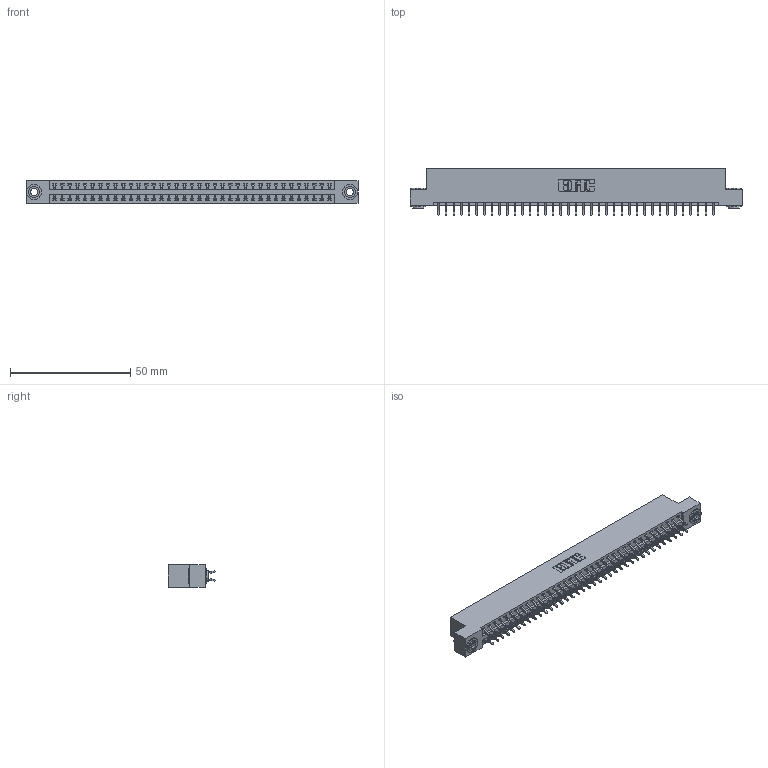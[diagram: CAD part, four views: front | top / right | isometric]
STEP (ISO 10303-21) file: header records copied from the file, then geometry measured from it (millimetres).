
FILE_DESCRIPTION (( 'STEP AP203' ), '1' );
FILE_NAME ('396-074-556-203.STEP', '2019-10-30T20:57:10', ( '' ), ( '' ), 'SwSTEP 2.0', 'SolidWorks 2016', '' );
FILE_SCHEMA (( 'CONFIG_CONTROL_DESIGN' ));
Length unit declared in the file: inch
Products named in the file (4): 396-074-556-203; 345-292-001_556 Tail; 345-250-002_345-250-002-102; 346 Part_Flush Mounting Lugs - 0.156 Dia-TH
Assembly tree (77 placements, depth 2):
  396-074-556-203
    346 Part_Flush Mounting Lugs - 0.156 Dia-TH
    345-292-001_556 Tail  x74
    345-250-002_345-250-002-102  x2
Bounding box: 138.05 x 19.57 x 9.4 mm (x, y, z)
Volume: 13439.1 mm3; surface area: 18539.8 mm2
Topology: 77 solids, 77 shells, 4452 faces, 13207 edges, 8702 vertices
Faces by surface type: plane 2972, cylinder 1472, cone 8
Entity records: 25690 total; most frequent: CARTESIAN_POINT 4231, ORIENTED_EDGE 4146, DIRECTION 3799, EDGE_CURVE 2073, VECTOR 1761, LINE 1761, VERTEX_POINT 1378, AXIS2_PLACEMENT_3D 1019
